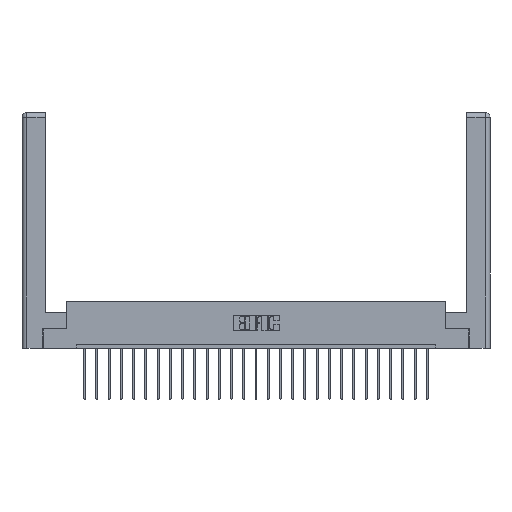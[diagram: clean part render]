
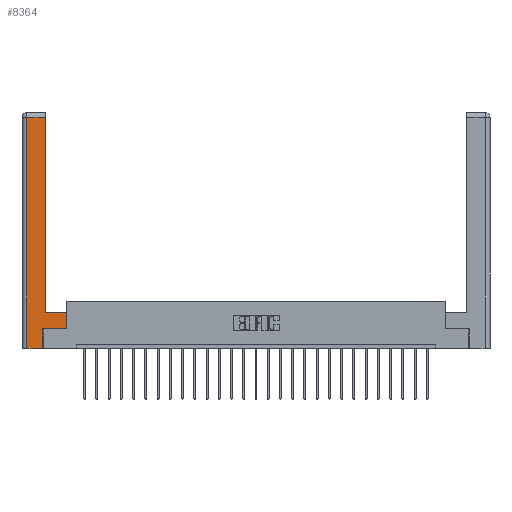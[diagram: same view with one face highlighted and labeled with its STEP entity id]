
A CAD part, top view. The second image highlights one B-rep face of the part: STEP entity #8364.
In plain terms, the highlighted planar face has unit normal (0, 0, 1).
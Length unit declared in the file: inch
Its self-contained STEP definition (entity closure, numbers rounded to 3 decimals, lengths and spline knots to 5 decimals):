
#1475 = ORIENTED_EDGE ( 'NONE', *, *, #11653, .T. ) ;
#1539 = VERTEX_POINT ( 'NONE', #2672 ) ;
#1687 = EDGE_CURVE ( 'NONE', #21489, #8502, #4272, .T. ) ;
#1696 = VECTOR ( 'NONE', #17013, 39.37008 ) ;
#2329 = LINE ( 'NONE', #15808, #8907 ) ;
#2492 = ORIENTED_EDGE ( 'NONE', *, *, #20881, .T. ) ;
#2500 = EDGE_CURVE ( 'NONE', #10375, #21489, #16765, .T. ) ;
#2672 = CARTESIAN_POINT ( 'NONE',  ( 0.565, 0.245, 0. ) ) ;
#2994 = CARTESIAN_POINT ( 'NONE',  ( 0.295, 3., 0. ) ) ;
#3338 = VECTOR ( 'NONE', #24583, 39.37008 ) ;
#3402 = ORIENTED_EDGE ( 'NONE', *, *, #1687, .T. ) ;
#4272 = LINE ( 'NONE', #4571, #3338 ) ;
#4326 = PLANE ( 'NONE',  #17174 ) ;
#4571 = CARTESIAN_POINT ( 'NONE',  ( 0.0615, 2.94, 0. ) ) ;
#4829 = LINE ( 'NONE', #10810, #1696 ) ;
#6033 = CARTESIAN_POINT ( 'NONE',  ( 0.265, 0.245, 0. ) ) ;
#8096 = DIRECTION ( 'NONE',  ( 1., 0., 0. ) ) ;
#8220 = DIRECTION ( 'NONE',  ( 0., -1., 0. ) ) ;
#8364 = ADVANCED_FACE ( 'NONE', ( #25663 ), #4326, .F. ) ;
#8407 = ORIENTED_EDGE ( 'NONE', *, *, #20744, .T. ) ;
#8502 = VERTEX_POINT ( 'NONE', #9133 ) ;
#8581 = CARTESIAN_POINT ( 'NONE',  ( 0.295, 0.45, 0. ) ) ;
#8907 = VECTOR ( 'NONE', #19572, 39.37008 ) ;
#9133 = CARTESIAN_POINT ( 'NONE',  ( 0.0615, 2.94, 0. ) ) ;
#10037 = EDGE_LOOP ( 'NONE', ( #23893, #3402, #8407, #13575, #2492, #1475, #16871, #13345 ) ) ;
#10241 = CARTESIAN_POINT ( 'NONE',  ( 0.295, 2.94, 0. ) ) ;
#10265 = CARTESIAN_POINT ( 'NONE',  ( 0.265, 0., 0. ) ) ;
#10375 = VERTEX_POINT ( 'NONE', #18663 ) ;
#10810 = CARTESIAN_POINT ( 'NONE',  ( 0.265, 0.245, 0. ) ) ;
#11653 = EDGE_CURVE ( 'NONE', #12790, #1539, #24950, .T. ) ;
#12003 = LINE ( 'NONE', #8581, #16974 ) ;
#12064 = VERTEX_POINT ( 'NONE', #16011 ) ;
#12292 = VERTEX_POINT ( 'NONE', #22763 ) ;
#12790 = VERTEX_POINT ( 'NONE', #6033 ) ;
#13345 = ORIENTED_EDGE ( 'NONE', *, *, #14981, .T. ) ;
#13407 = LINE ( 'NONE', #10265, #20916 ) ;
#13575 = ORIENTED_EDGE ( 'NONE', *, *, #23480, .T. ) ;
#14055 = CARTESIAN_POINT ( 'NONE',  ( 0.565, 0.45, 0. ) ) ;
#14141 = CARTESIAN_POINT ( 'NONE',  ( 0.0615, 0., 0. ) ) ;
#14981 = EDGE_CURVE ( 'NONE', #19050, #10375, #12003, .T. ) ;
#15501 = VECTOR ( 'NONE', #22831, 39.37008 ) ;
#15808 = CARTESIAN_POINT ( 'NONE',  ( 0.565, 0.45, 0. ) ) ;
#16011 = CARTESIAN_POINT ( 'NONE',  ( 0.0615, 0., 0. ) ) ;
#16765 = LINE ( 'NONE', #2994, #15501 ) ;
#16871 = ORIENTED_EDGE ( 'NONE', *, *, #25561, .T. ) ;
#16974 = VECTOR ( 'NONE', #20733, 39.37008 ) ;
#17013 = DIRECTION ( 'NONE',  ( 0., 1., 0. ) ) ;
#17174 = AXIS2_PLACEMENT_3D ( 'NONE', #22009, #22757, #22916 ) ;
#18053 = VECTOR ( 'NONE', #8220, 39.37008 ) ;
#18657 = LINE ( 'NONE', #14141, #18053 ) ;
#18663 = CARTESIAN_POINT ( 'NONE',  ( 0.295, 0.45, 0. ) ) ;
#19050 = VERTEX_POINT ( 'NONE', #14055 ) ;
#19572 = DIRECTION ( 'NONE',  ( 0., 1., 0. ) ) ;
#19985 = CARTESIAN_POINT ( 'NONE',  ( 0.565, 0.245, 0. ) ) ;
#20733 = DIRECTION ( 'NONE',  ( -1., 0., 0. ) ) ;
#20744 = EDGE_CURVE ( 'NONE', #8502, #12064, #18657, .T. ) ;
#20881 = EDGE_CURVE ( 'NONE', #12292, #12790, #4829, .T. ) ;
#20916 = VECTOR ( 'NONE', #25893, 39.37008 ) ;
#21489 = VERTEX_POINT ( 'NONE', #10241 ) ;
#22009 = CARTESIAN_POINT ( 'NONE',  ( 0., 0., 0. ) ) ;
#22757 = DIRECTION ( 'NONE',  ( 0., 0., -1. ) ) ;
#22763 = CARTESIAN_POINT ( 'NONE',  ( 0.265, 0., 0. ) ) ;
#22831 = DIRECTION ( 'NONE',  ( 0., 1., 0. ) ) ;
#22916 = DIRECTION ( 'NONE',  ( -1., 0., 0. ) ) ;
#23404 = VECTOR ( 'NONE', #8096, 39.37008 ) ;
#23480 = EDGE_CURVE ( 'NONE', #12064, #12292, #13407, .T. ) ;
#23893 = ORIENTED_EDGE ( 'NONE', *, *, #2500, .T. ) ;
#24583 = DIRECTION ( 'NONE',  ( -1., 0., 0. ) ) ;
#24950 = LINE ( 'NONE', #19985, #23404 ) ;
#25561 = EDGE_CURVE ( 'NONE', #1539, #19050, #2329, .T. ) ;
#25663 = FACE_OUTER_BOUND ( 'NONE', #10037, .T. ) ;
#25893 = DIRECTION ( 'NONE',  ( 1., 0., 0. ) ) ;
